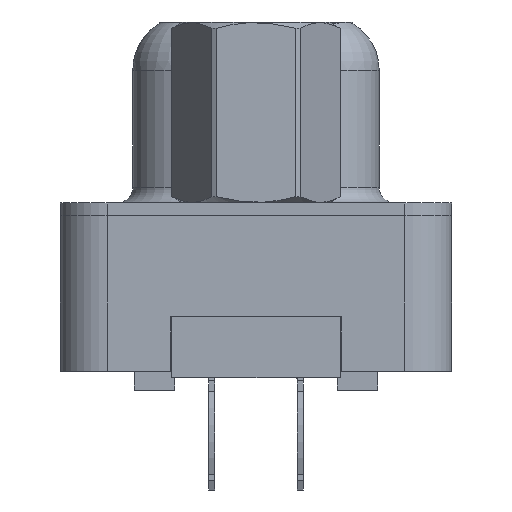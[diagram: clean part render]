
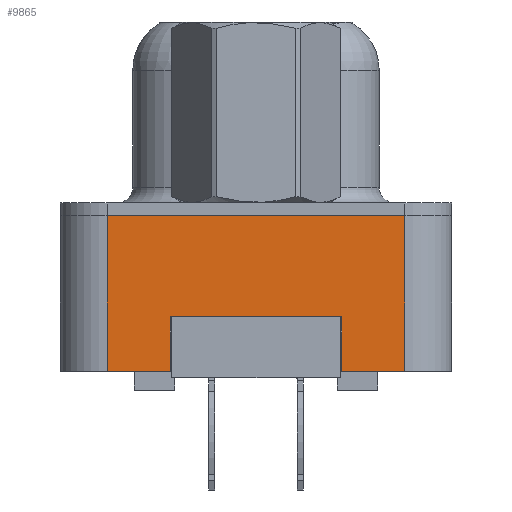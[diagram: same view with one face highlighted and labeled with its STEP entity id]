
A CAD part, left-side view. The second image highlights one B-rep face of the part: STEP entity #9865.
In plain terms, the highlighted planar face has unit normal (-1, 0, 0).
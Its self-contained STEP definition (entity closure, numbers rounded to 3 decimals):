
#496 = LINE ( 'NONE', #16790, #14913 ) ;
#623 = CARTESIAN_POINT ( 'NONE',  ( -2.945, 2.75, -3.25 ) ) ;
#971 = CARTESIAN_POINT ( 'NONE',  ( -2.945, -4.775, -5. ) ) ;
#1577 = PLANE ( 'NONE',  #2315 ) ;
#1790 = DIRECTION ( 'NONE',  ( 0., 0., 1. ) ) ;
#2315 = AXIS2_PLACEMENT_3D ( 'NONE', #12033, #23029, #8838 ) ;
#2511 = ORIENTED_EDGE ( 'NONE', *, *, #19263, .T. ) ;
#2756 = LINE ( 'NONE', #4416, #17521 ) ;
#2892 = FACE_OUTER_BOUND ( 'NONE', #14169, .T. ) ;
#3821 = VERTEX_POINT ( 'NONE', #14139 ) ;
#3857 = ORIENTED_EDGE ( 'NONE', *, *, #12392, .F. ) ;
#3882 = VERTEX_POINT ( 'NONE', #19752 ) ;
#4217 = VECTOR ( 'NONE', #17216, 1000. ) ;
#4408 = CARTESIAN_POINT ( 'NONE',  ( -2.945, -2.75, -3.25 ) ) ;
#4416 = CARTESIAN_POINT ( 'NONE',  ( -2.945, -4.775, -5. ) ) ;
#4872 = ORIENTED_EDGE ( 'NONE', *, *, #14642, .T. ) ;
#6267 = DIRECTION ( 'NONE',  ( 0., -1., 0. ) ) ;
#6374 = LINE ( 'NONE', #20575, #11485 ) ;
#7559 = EDGE_CURVE ( 'NONE', #11193, #15496, #13860, .T. ) ;
#7662 = ORIENTED_EDGE ( 'NONE', *, *, #19216, .F. ) ;
#7905 = ORIENTED_EDGE ( 'NONE', *, *, #14765, .T. ) ;
#7979 = DIRECTION ( 'NONE',  ( 0., -1., 0. ) ) ;
#8297 = EDGE_CURVE ( 'NONE', #3821, #15496, #16176, .T. ) ;
#8357 = ORIENTED_EDGE ( 'NONE', *, *, #21866, .F. ) ;
#8527 = CARTESIAN_POINT ( 'NONE',  ( -2.945, -2.75, -5. ) ) ;
#8838 = DIRECTION ( 'NONE',  ( 0., 0., 1. ) ) ;
#9173 = LINE ( 'NONE', #623, #17899 ) ;
#9865 = ADVANCED_FACE ( 'NONE', ( #2892 ), #1577, .T. ) ;
#10924 = DIRECTION ( 'NONE',  ( 0., 0., 1. ) ) ;
#11193 = VERTEX_POINT ( 'NONE', #12217 ) ;
#11485 = VECTOR ( 'NONE', #6267, 1000. ) ;
#12033 = CARTESIAN_POINT ( 'NONE',  ( -2.945, -4.775, -5. ) ) ;
#12057 = VERTEX_POINT ( 'NONE', #971 ) ;
#12217 = CARTESIAN_POINT ( 'NONE',  ( -2.945, 4.775, -5. ) ) ;
#12392 = EDGE_CURVE ( 'NONE', #11193, #19414, #20014, .T. ) ;
#13398 = VECTOR ( 'NONE', #18824, 1000. ) ;
#13860 = LINE ( 'NONE', #21026, #4217 ) ;
#14139 = CARTESIAN_POINT ( 'NONE',  ( -2.945, 2.75, -3.25 ) ) ;
#14169 = EDGE_LOOP ( 'NONE', ( #7905, #2511, #4872, #8357, #3857, #21109, #21394, #7662 ) ) ;
#14642 = EDGE_CURVE ( 'NONE', #12057, #18101, #496, .T. ) ;
#14765 = EDGE_CURVE ( 'NONE', #3882, #23120, #22383, .T. ) ;
#14913 = VECTOR ( 'NONE', #10924, 1000. ) ;
#15496 = VERTEX_POINT ( 'NONE', #19625 ) ;
#16176 = LINE ( 'NONE', #16285, #22353 ) ;
#16285 = CARTESIAN_POINT ( 'NONE',  ( -2.945, 2.75, -3.25 ) ) ;
#16506 = CARTESIAN_POINT ( 'NONE',  ( -2.945, 4.775, 0. ) ) ;
#16790 = CARTESIAN_POINT ( 'NONE',  ( -2.945, -4.775, -5. ) ) ;
#17216 = DIRECTION ( 'NONE',  ( 0., -1., 0. ) ) ;
#17521 = VECTOR ( 'NONE', #7979, 1000. ) ;
#17899 = VECTOR ( 'NONE', #20277, 1000. ) ;
#18101 = VERTEX_POINT ( 'NONE', #19380 ) ;
#18193 = DIRECTION ( 'NONE',  ( 0., 0., -1. ) ) ;
#18824 = DIRECTION ( 'NONE',  ( 0., 0., -1. ) ) ;
#19216 = EDGE_CURVE ( 'NONE', #3882, #3821, #9173, .T. ) ;
#19263 = EDGE_CURVE ( 'NONE', #23120, #12057, #2756, .T. ) ;
#19380 = CARTESIAN_POINT ( 'NONE',  ( -2.945, -4.775, 0. ) ) ;
#19414 = VERTEX_POINT ( 'NONE', #16506 ) ;
#19625 = CARTESIAN_POINT ( 'NONE',  ( -2.945, 2.75, -5. ) ) ;
#19752 = CARTESIAN_POINT ( 'NONE',  ( -2.945, -2.75, -3.25 ) ) ;
#19904 = CARTESIAN_POINT ( 'NONE',  ( -2.945, 4.775, -5. ) ) ;
#20014 = LINE ( 'NONE', #19904, #22860 ) ;
#20277 = DIRECTION ( 'NONE',  ( 0., 1., 0. ) ) ;
#20575 = CARTESIAN_POINT ( 'NONE',  ( -2.945, -4.775, 0. ) ) ;
#21026 = CARTESIAN_POINT ( 'NONE',  ( -2.945, -4.775, -5. ) ) ;
#21109 = ORIENTED_EDGE ( 'NONE', *, *, #7559, .T. ) ;
#21394 = ORIENTED_EDGE ( 'NONE', *, *, #8297, .F. ) ;
#21866 = EDGE_CURVE ( 'NONE', #19414, #18101, #6374, .T. ) ;
#22353 = VECTOR ( 'NONE', #18193, 1000. ) ;
#22383 = LINE ( 'NONE', #4408, #13398 ) ;
#22860 = VECTOR ( 'NONE', #1790, 1000. ) ;
#23029 = DIRECTION ( 'NONE',  ( -1., 0., 0. ) ) ;
#23120 = VERTEX_POINT ( 'NONE', #8527 ) ;
